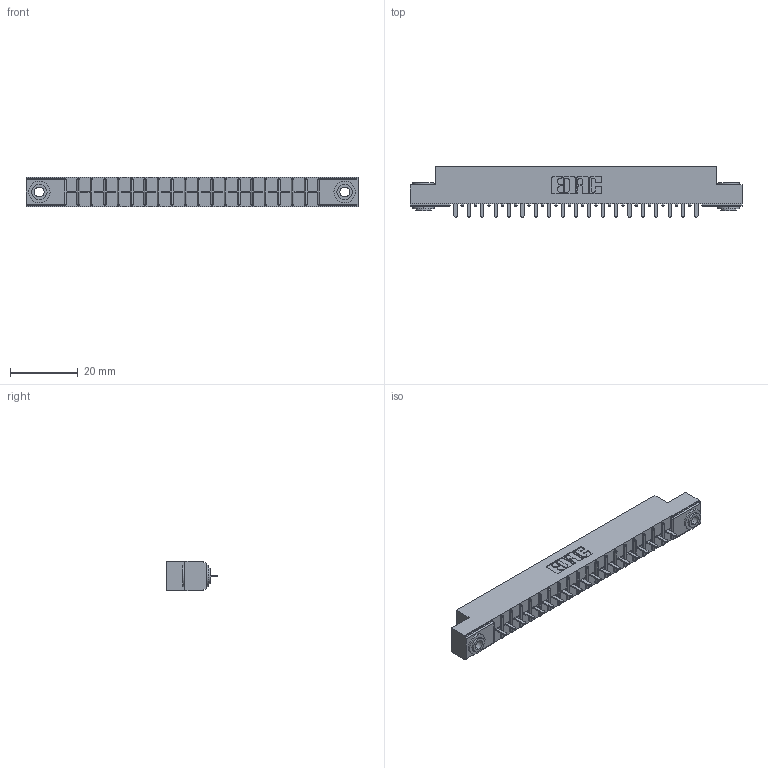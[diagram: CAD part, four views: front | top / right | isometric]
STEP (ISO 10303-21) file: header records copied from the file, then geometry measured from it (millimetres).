
FILE_DESCRIPTION (( 'STEP AP203' ), '1' );
FILE_NAME ('316-019-521-103.STEP', '2018-07-31T01:28:27', ( '' ), ( '' ), 'SwSTEP 2.0', 'SolidWorks 2016', '' );
FILE_SCHEMA (( 'CONFIG_CONTROL_DESIGN' ));
Length unit declared in the file: inch
Products named in the file (4): 306 Part_.156 Dia; 306-290-001_121; 345-250-002_345-250-002-102; 316-019-521-103
Assembly tree (22 placements, depth 2):
  316-019-521-103
    306 Part_.156 Dia
    306-290-001_121  x19
    345-250-002_345-250-002-102  x2
Bounding box: 98.3 x 14.88 x 8.71 mm (x, y, z)
Volume: 6690.4 mm3; surface area: 9908.6 mm2
Topology: 22 solids, 22 shells, 1498 faces, 4171 edges, 2674 vertices
Faces by surface type: plane 985, cylinder 429, sphere 76, cone 8
Entity records: 21719 total; most frequent: CARTESIAN_POINT 3621, DIRECTION 3587, ORIENTED_EDGE 3578, EDGE_CURVE 1789, LINE 1379, VECTOR 1379, VERTEX_POINT 1138, AXIS2_PLACEMENT_3D 1104
